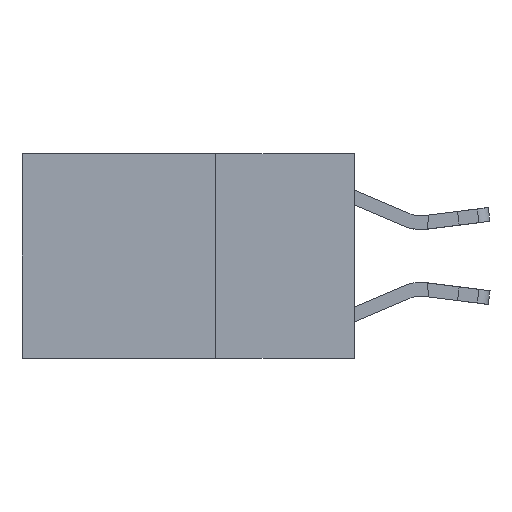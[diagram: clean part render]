
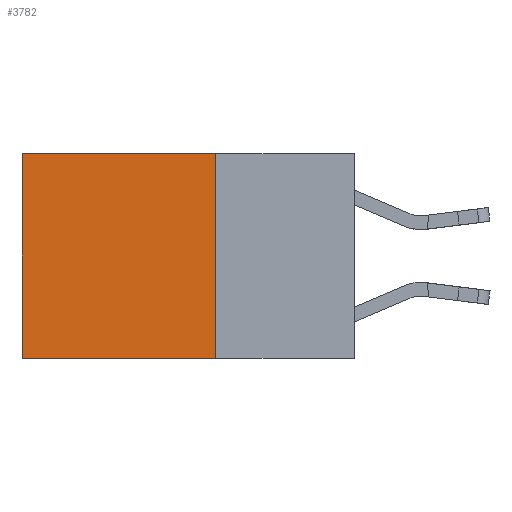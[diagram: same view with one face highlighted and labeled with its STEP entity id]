
A CAD part, left-side view. The second image highlights one B-rep face of the part: STEP entity #3782.
In plain terms, the highlighted planar face has unit normal (-1, 0, 0).
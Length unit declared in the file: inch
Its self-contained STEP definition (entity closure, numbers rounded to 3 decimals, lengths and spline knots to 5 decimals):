
#330 = LINE ( 'NONE', #4789, #11577 ) ;
#985 = CARTESIAN_POINT ( 'NONE',  ( 0.2625, 0.25, 0. ) ) ;
#2220 = ORIENTED_EDGE ( 'NONE', *, *, #18406, .T. ) ;
#2528 = LINE ( 'NONE', #21551, #24835 ) ;
#2915 = DIRECTION ( 'NONE',  ( 0., 1., 0. ) ) ;
#3661 = ORIENTED_EDGE ( 'NONE', *, *, #24801, .T. ) ;
#3782 = ADVANCED_FACE ( 'NONE', ( #13679 ), #12740, .F. ) ;
#4789 = CARTESIAN_POINT ( 'NONE',  ( 0.2625, 0.6, 0. ) ) ;
#5407 = VERTEX_POINT ( 'NONE', #21359 ) ;
#6001 = VERTEX_POINT ( 'NONE', #23981 ) ;
#6551 = DIRECTION ( 'NONE',  ( 0., 0., -1. ) ) ;
#7315 = CARTESIAN_POINT ( 'NONE',  ( 0.2625, 0.25, 0. ) ) ;
#8035 = DIRECTION ( 'NONE',  ( 0., 1., 0. ) ) ;
#9719 = DIRECTION ( 'NONE',  ( 0., 0., -1. ) ) ;
#10658 = DIRECTION ( 'NONE',  ( 1., 0., 0. ) ) ;
#10660 = EDGE_CURVE ( 'NONE', #6001, #5407, #17132, .T. ) ;
#11577 = VECTOR ( 'NONE', #20602, 39.37008 ) ;
#11914 = EDGE_LOOP ( 'NONE', ( #3661, #12512, #15556, #2220 ) ) ;
#12512 = ORIENTED_EDGE ( 'NONE', *, *, #10660, .F. ) ;
#12740 = PLANE ( 'NONE',  #15708 ) ;
#12916 = CARTESIAN_POINT ( 'NONE',  ( 0.2625, 0.25, 0. ) ) ;
#13679 = FACE_OUTER_BOUND ( 'NONE', #11914, .T. ) ;
#14538 = VERTEX_POINT ( 'NONE', #16222 ) ;
#15556 = ORIENTED_EDGE ( 'NONE', *, *, #25018, .F. ) ;
#15693 = VECTOR ( 'NONE', #2915, 39.37008 ) ;
#15708 = AXIS2_PLACEMENT_3D ( 'NONE', #12916, #10658, #6551 ) ;
#16222 = CARTESIAN_POINT ( 'NONE',  ( 0.2625, 0.6, 0. ) ) ;
#16612 = LINE ( 'NONE', #985, #15693 ) ;
#17132 = LINE ( 'NONE', #23776, #18973 ) ;
#18406 = EDGE_CURVE ( 'NONE', #22789, #14538, #16612, .T. ) ;
#18973 = VECTOR ( 'NONE', #8035, 39.37008 ) ;
#20602 = DIRECTION ( 'NONE',  ( 0., 0., -1. ) ) ;
#21359 = CARTESIAN_POINT ( 'NONE',  ( 0.2625, 0.6, -0.37 ) ) ;
#21551 = CARTESIAN_POINT ( 'NONE',  ( 0.2625, 0.25, 0. ) ) ;
#22789 = VERTEX_POINT ( 'NONE', #7315 ) ;
#23776 = CARTESIAN_POINT ( 'NONE',  ( 0.2625, 0.25, -0.37 ) ) ;
#23981 = CARTESIAN_POINT ( 'NONE',  ( 0.2625, 0.25, -0.37 ) ) ;
#24801 = EDGE_CURVE ( 'NONE', #14538, #5407, #330, .T. ) ;
#24835 = VECTOR ( 'NONE', #9719, 39.37008 ) ;
#25018 = EDGE_CURVE ( 'NONE', #22789, #6001, #2528, .T. ) ;
